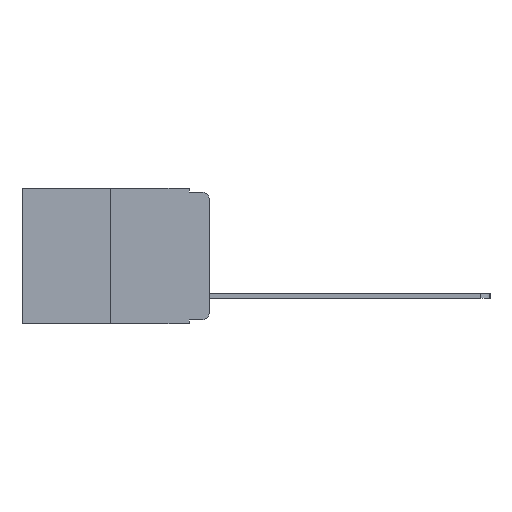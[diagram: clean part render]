
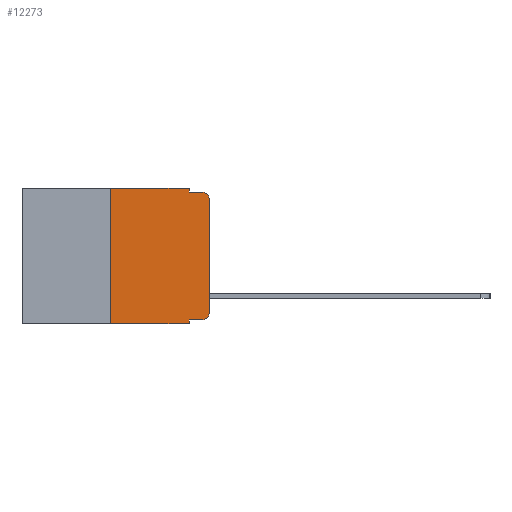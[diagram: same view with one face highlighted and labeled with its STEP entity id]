
A CAD part, left-side view. The second image highlights one B-rep face of the part: STEP entity #12273.
In plain terms, the highlighted planar face has unit normal (-1, 0, 0).
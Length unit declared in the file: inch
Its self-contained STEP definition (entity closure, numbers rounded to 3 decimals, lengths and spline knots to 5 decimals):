
#63 = VERTEX_POINT ( 'NONE', #6281 ) ;
#271 = CARTESIAN_POINT ( 'NONE',  ( 0., 0., 0. ) ) ;
#705 = EDGE_CURVE ( 'NONE', #848, #10356, #9113, .T. ) ;
#746 = VERTEX_POINT ( 'NONE', #2838 ) ;
#771 = ORIENTED_EDGE ( 'NONE', *, *, #9377, .T. ) ;
#842 = VECTOR ( 'NONE', #1211, 39.37008 ) ;
#848 = VERTEX_POINT ( 'NONE', #10021 ) ;
#1211 = DIRECTION ( 'NONE',  ( 0., -1., 0. ) ) ;
#1395 = VERTEX_POINT ( 'NONE', #15084 ) ;
#1610 = DIRECTION ( 'NONE',  ( 0., 0., 1. ) ) ;
#1923 = VECTOR ( 'NONE', #5724, 39.37008 ) ;
#2012 = ORIENTED_EDGE ( 'NONE', *, *, #4206, .F. ) ;
#2051 = CARTESIAN_POINT ( 'NONE',  ( 0., 0.02, -0.333 ) ) ;
#2102 = FACE_OUTER_BOUND ( 'NONE', #7360, .T. ) ;
#2415 = ORIENTED_EDGE ( 'NONE', *, *, #2467, .F. ) ;
#2467 = EDGE_CURVE ( 'NONE', #848, #8882, #5044, .T. ) ;
#2838 = CARTESIAN_POINT ( 'NONE',  ( 0., 0., -0.313 ) ) ;
#2898 = CARTESIAN_POINT ( 'NONE',  ( 0., 0.051, -0.333 ) ) ;
#2914 = AXIS2_PLACEMENT_3D ( 'NONE', #5773, #14510, #7098 ) ;
#3069 = LINE ( 'NONE', #11204, #9512 ) ;
#3072 = VECTOR ( 'NONE', #12107, 39.37008 ) ;
#3853 = CIRCLE ( 'NONE', #10787, 0.02 ) ;
#4206 = EDGE_CURVE ( 'NONE', #8557, #9841, #11717, .T. ) ;
#4245 = ORIENTED_EDGE ( 'NONE', *, *, #8562, .T. ) ;
#5044 = LINE ( 'NONE', #12665, #11037 ) ;
#5073 = DIRECTION ( 'NONE',  ( 1., 0., 0. ) ) ;
#5544 = VERTEX_POINT ( 'NONE', #15685 ) ;
#5724 = DIRECTION ( 'NONE',  ( 0., 0., 1. ) ) ;
#5773 = CARTESIAN_POINT ( 'NONE',  ( 0., 0.02, -0.313 ) ) ;
#5865 = EDGE_CURVE ( 'NONE', #8557, #8882, #10744, .T. ) ;
#5890 = ORIENTED_EDGE ( 'NONE', *, *, #705, .T. ) ;
#5973 = DIRECTION ( 'NONE',  ( 0., 0., -1. ) ) ;
#6281 = CARTESIAN_POINT ( 'NONE',  ( 0., 0.051, -0.01 ) ) ;
#6301 = CARTESIAN_POINT ( 'NONE',  ( 0., 0.02, -0.03 ) ) ;
#6396 = CARTESIAN_POINT ( 'NONE',  ( 0., 0.473, 0. ) ) ;
#6423 = LINE ( 'NONE', #6396, #15926 ) ;
#6430 = CARTESIAN_POINT ( 'NONE',  ( 0., 0.25, 0. ) ) ;
#6451 = CARTESIAN_POINT ( 'NONE',  ( 0., 0.25, 0. ) ) ;
#6531 = LINE ( 'NONE', #7148, #3072 ) ;
#6832 = EDGE_CURVE ( 'NONE', #1395, #63, #3069, .T. ) ;
#7098 = DIRECTION ( 'NONE',  ( 0., 0., -1. ) ) ;
#7148 = CARTESIAN_POINT ( 'NONE',  ( 0., 0.051, -0.01 ) ) ;
#7297 = LINE ( 'NONE', #271, #8500 ) ;
#7360 = EDGE_LOOP ( 'NONE', ( #771, #4245, #14287, #8108, #15045, #2012, #15418, #2415, #5890, #9686 ) ) ;
#7614 = DIRECTION ( 'NONE',  ( 0., 0., -1. ) ) ;
#7709 = EDGE_CURVE ( 'NONE', #63, #8428, #6531, .T. ) ;
#8108 = ORIENTED_EDGE ( 'NONE', *, *, #6832, .F. ) ;
#8428 = VERTEX_POINT ( 'NONE', #13534 ) ;
#8500 = VECTOR ( 'NONE', #1610, 39.37008 ) ;
#8557 = VERTEX_POINT ( 'NONE', #16163 ) ;
#8562 = EDGE_CURVE ( 'NONE', #5544, #8428, #3853, .T. ) ;
#8722 = VECTOR ( 'NONE', #15743, 39.37008 ) ;
#8733 = DIRECTION ( 'NONE',  ( 0., 0., -1. ) ) ;
#8882 = VERTEX_POINT ( 'NONE', #13251 ) ;
#8976 = DIRECTION ( 'NONE',  ( 0., -1., 0. ) ) ;
#9113 = LINE ( 'NONE', #2898, #8722 ) ;
#9377 = EDGE_CURVE ( 'NONE', #746, #5544, #7297, .T. ) ;
#9512 = VECTOR ( 'NONE', #8733, 39.37008 ) ;
#9686 = ORIENTED_EDGE ( 'NONE', *, *, #16259, .T. ) ;
#9841 = VERTEX_POINT ( 'NONE', #6430 ) ;
#10021 = CARTESIAN_POINT ( 'NONE',  ( 0., 0.051, -0.333 ) ) ;
#10356 = VERTEX_POINT ( 'NONE', #2051 ) ;
#10744 = LINE ( 'NONE', #16320, #842 ) ;
#10787 = AXIS2_PLACEMENT_3D ( 'NONE', #6301, #15003, #7614 ) ;
#11037 = VECTOR ( 'NONE', #5973, 39.37008 ) ;
#11204 = CARTESIAN_POINT ( 'NONE',  ( 0., 0.051, 0. ) ) ;
#11717 = LINE ( 'NONE', #6451, #1923 ) ;
#11718 = AXIS2_PLACEMENT_3D ( 'NONE', #15021, #5073, #13852 ) ;
#12107 = DIRECTION ( 'NONE',  ( 0., -1., 0. ) ) ;
#12273 = ADVANCED_FACE ( 'NONE', ( #2102 ), #12629, .F. ) ;
#12629 = PLANE ( 'NONE',  #11718 ) ;
#12665 = CARTESIAN_POINT ( 'NONE',  ( 0., 0.051, 0. ) ) ;
#13251 = CARTESIAN_POINT ( 'NONE',  ( 0., 0.051, -0.343 ) ) ;
#13534 = CARTESIAN_POINT ( 'NONE',  ( 0., 0.02, -0.01 ) ) ;
#13852 = DIRECTION ( 'NONE',  ( 0., 0., -1. ) ) ;
#14287 = ORIENTED_EDGE ( 'NONE', *, *, #7709, .F. ) ;
#14460 = EDGE_CURVE ( 'NONE', #9841, #1395, #6423, .T. ) ;
#14510 = DIRECTION ( 'NONE',  ( -1., 0., 0. ) ) ;
#15003 = DIRECTION ( 'NONE',  ( -1., 0., 0. ) ) ;
#15021 = CARTESIAN_POINT ( 'NONE',  ( 0., 0.473, 0. ) ) ;
#15045 = ORIENTED_EDGE ( 'NONE', *, *, #14460, .F. ) ;
#15084 = CARTESIAN_POINT ( 'NONE',  ( 0., 0.051, 0. ) ) ;
#15418 = ORIENTED_EDGE ( 'NONE', *, *, #5865, .T. ) ;
#15685 = CARTESIAN_POINT ( 'NONE',  ( 0., 0., -0.03 ) ) ;
#15743 = DIRECTION ( 'NONE',  ( 0., -1., 0. ) ) ;
#15926 = VECTOR ( 'NONE', #8976, 39.37008 ) ;
#16045 = CIRCLE ( 'NONE', #2914, 0.02 ) ;
#16163 = CARTESIAN_POINT ( 'NONE',  ( 0., 0.25, -0.343 ) ) ;
#16259 = EDGE_CURVE ( 'NONE', #10356, #746, #16045, .T. ) ;
#16320 = CARTESIAN_POINT ( 'NONE',  ( 0., 0.473, -0.343 ) ) ;
